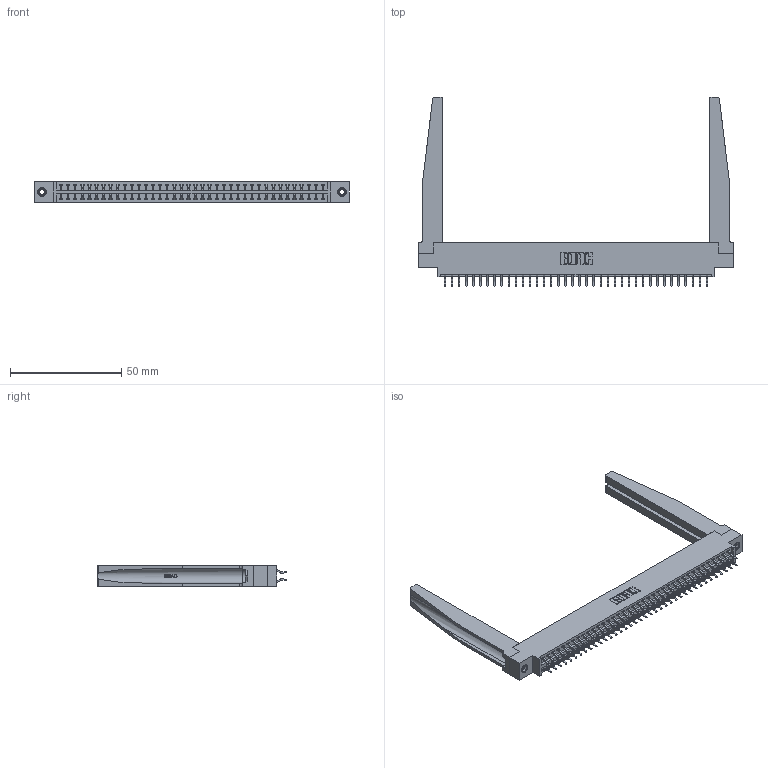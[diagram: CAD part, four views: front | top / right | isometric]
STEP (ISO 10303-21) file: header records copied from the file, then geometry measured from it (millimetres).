
FILE_DESCRIPTION (( 'STEP AP203' ), '1' );
FILE_NAME ('346-076-556-878.STEP', '2022-05-25T12:56:57', ( '' ), ( '' ), 'SwSTEP 2.0', 'SolidWorks 2020', '' );
FILE_SCHEMA (( 'CONFIG_CONTROL_DESIGN' ));
Length unit declared in the file: inch
Products named in the file (5): 345-292-001_556 Tail; 346-076-556-878; 346 Part_0.170 Offset - 0.156 Dia-TH; 345-250-001_345-250-001-102; 346-220-078_345-220-078
Assembly tree (81 placements, depth 2):
  346-076-556-878
    346 Part_0.170 Offset - 0.156 Dia-TH
    345-292-001_556 Tail  x76
    346-220-078_345-220-078  x2
    345-250-001_345-250-001-102  x2
Bounding box: 141.22 x 84.84 x 9.4 mm (x, y, z)
Volume: 20473.2 mm3; surface area: 25263.3 mm2
Topology: 81 solids, 81 shells, 4782 faces, 14133 edges, 9310 vertices
Faces by surface type: plane 3200, cylinder 1530, bspline 36, cone 12, torus 4
Entity records: 30854 total; most frequent: CARTESIAN_POINT 6049, ORIENTED_EDGE 4858, DIRECTION 4355, EDGE_CURVE 2429, LINE 2043, VECTOR 2043, VERTEX_POINT 1612, AXIS2_PLACEMENT_3D 1156
